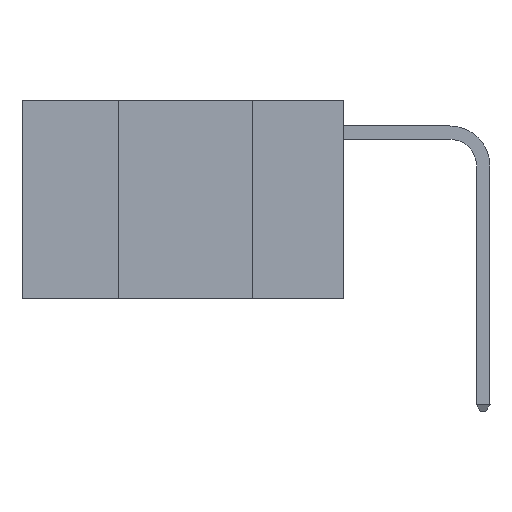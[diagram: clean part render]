
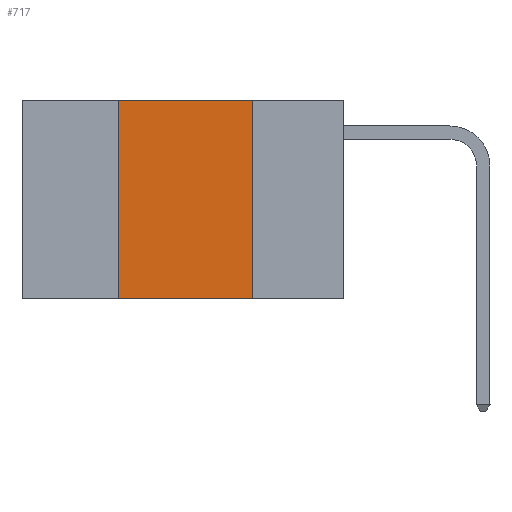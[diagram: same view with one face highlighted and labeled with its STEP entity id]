
A CAD part, left-side view. The second image highlights one B-rep face of the part: STEP entity #717.
In plain terms, the highlighted planar face has unit normal (-1, 0, 0).
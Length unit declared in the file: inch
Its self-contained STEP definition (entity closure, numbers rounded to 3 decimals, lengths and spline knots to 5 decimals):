
#27 = EDGE_LOOP ( 'NONE', ( #11583, #12413, #6532, #6922 ) ) ;
#380 = CARTESIAN_POINT ( 'NONE',  ( 0., 0.17, -0.37 ) ) ;
#635 = LINE ( 'NONE', #3939, #10336 ) ;
#717 = ADVANCED_FACE ( 'NONE', ( #11264 ), #13325, .F. ) ;
#1158 = EDGE_CURVE ( 'NONE', #14834, #7193, #14554, .T. ) ;
#1321 = CARTESIAN_POINT ( 'NONE',  ( 0., 0.42, 0. ) ) ;
#2518 = LINE ( 'NONE', #14553, #8816 ) ;
#2616 = EDGE_CURVE ( 'NONE', #14834, #15539, #2518, .T. ) ;
#3460 = EDGE_CURVE ( 'NONE', #9139, #15539, #12152, .T. ) ;
#3939 = CARTESIAN_POINT ( 'NONE',  ( 0., 0.6, 0. ) ) ;
#5754 = CARTESIAN_POINT ( 'NONE',  ( 0., 0.17, 0. ) ) ;
#6159 = DIRECTION ( 'NONE',  ( 0., 0., -1. ) ) ;
#6532 = ORIENTED_EDGE ( 'NONE', *, *, #1158, .F. ) ;
#6707 = CARTESIAN_POINT ( 'NONE',  ( 0., 0.6, 0. ) ) ;
#6738 = CARTESIAN_POINT ( 'NONE',  ( 0., 0.42, 0. ) ) ;
#6922 = ORIENTED_EDGE ( 'NONE', *, *, #2616, .T. ) ;
#7193 = VERTEX_POINT ( 'NONE', #6738 ) ;
#7902 = VECTOR ( 'NONE', #12019, 39.37008 ) ;
#8816 = VECTOR ( 'NONE', #12934, 39.37008 ) ;
#8947 = DIRECTION ( 'NONE',  ( 0., -1., 0. ) ) ;
#9139 = VERTEX_POINT ( 'NONE', #5754 ) ;
#10336 = VECTOR ( 'NONE', #8947, 39.37008 ) ;
#11264 = FACE_OUTER_BOUND ( 'NONE', #27, .T. ) ;
#11583 = ORIENTED_EDGE ( 'NONE', *, *, #3460, .F. ) ;
#12019 = DIRECTION ( 'NONE',  ( 0., 0., 1. ) ) ;
#12152 = LINE ( 'NONE', #13418, #16195 ) ;
#12356 = AXIS2_PLACEMENT_3D ( 'NONE', #6707, #12913, #14276 ) ;
#12413 = ORIENTED_EDGE ( 'NONE', *, *, #16028, .F. ) ;
#12913 = DIRECTION ( 'NONE',  ( 1., 0., 0. ) ) ;
#12934 = DIRECTION ( 'NONE',  ( 0., -1., 0. ) ) ;
#13275 = CARTESIAN_POINT ( 'NONE',  ( 0., 0.42, -0.37 ) ) ;
#13325 = PLANE ( 'NONE',  #12356 ) ;
#13418 = CARTESIAN_POINT ( 'NONE',  ( 0., 0.17, 0. ) ) ;
#14276 = DIRECTION ( 'NONE',  ( 0., 0., -1. ) ) ;
#14553 = CARTESIAN_POINT ( 'NONE',  ( 0., 0.6, -0.37 ) ) ;
#14554 = LINE ( 'NONE', #1321, #7902 ) ;
#14834 = VERTEX_POINT ( 'NONE', #13275 ) ;
#15539 = VERTEX_POINT ( 'NONE', #380 ) ;
#16028 = EDGE_CURVE ( 'NONE', #7193, #9139, #635, .T. ) ;
#16195 = VECTOR ( 'NONE', #6159, 39.37008 ) ;
